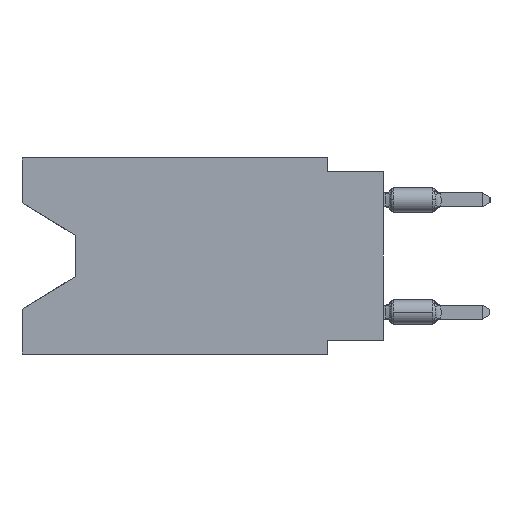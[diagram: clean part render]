
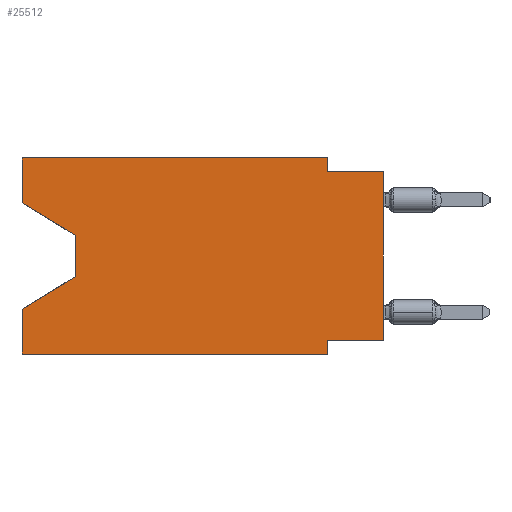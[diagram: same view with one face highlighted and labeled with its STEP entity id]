
A CAD part, left-side view. The second image highlights one B-rep face of the part: STEP entity #25512.
In plain terms, the highlighted planar face has unit normal (-1, 0, 0).
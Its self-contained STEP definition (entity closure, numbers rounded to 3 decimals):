
#20 = CARTESIAN_POINT ( 'NONE',  ( 0., 0., 0. ) ) ;
#696 = AXIS2_PLACEMENT_3D ( 'NONE', #6704, #10445, #43585 ) ;
#1336 = LINE ( 'NONE', #41915, #28280 ) ;
#2586 = VERTEX_POINT ( 'NONE', #45699 ) ;
#2714 = VERTEX_POINT ( 'NONE', #10147 ) ;
#3688 = VECTOR ( 'NONE', #42224, 1000. ) ;
#3750 = VECTOR ( 'NONE', #26880, 1000. ) ;
#3807 = EDGE_CURVE ( 'NONE', #29606, #2586, #11725, .T. ) ;
#5046 = LINE ( 'NONE', #40868, #29410 ) ;
#5248 = VECTOR ( 'NONE', #26307, 1000. ) ;
#5358 = VERTEX_POINT ( 'NONE', #15399 ) ;
#5887 = DIRECTION ( 'NONE',  ( 0., -1., 0. ) ) ;
#6704 = CARTESIAN_POINT ( 'NONE',  ( 0., 16.383, 0. ) ) ;
#6918 = ORIENTED_EDGE ( 'NONE', *, *, #27412, .F. ) ;
#7572 = ORIENTED_EDGE ( 'NONE', *, *, #3807, .T. ) ;
#9742 = VERTEX_POINT ( 'NONE', #44447 ) ;
#9893 = CARTESIAN_POINT ( 'NONE',  ( 0., 16.383, -8.89 ) ) ;
#10123 = CARTESIAN_POINT ( 'NONE',  ( 0., 0., -0.635 ) ) ;
#10147 = CARTESIAN_POINT ( 'NONE',  ( 0., 0., -8.255 ) ) ;
#10445 = DIRECTION ( 'NONE',  ( 1., 0., 0. ) ) ;
#11347 = CARTESIAN_POINT ( 'NONE',  ( 0., 16.383, -2.038 ) ) ;
#11725 = LINE ( 'NONE', #23680, #15605 ) ;
#12959 = LINE ( 'NONE', #29158, #32924 ) ;
#14047 = EDGE_CURVE ( 'NONE', #5358, #40531, #46461, .T. ) ;
#14627 = VECTOR ( 'NONE', #35396, 1000. ) ;
#14954 = EDGE_CURVE ( 'NONE', #45347, #30562, #18975, .T. ) ;
#15399 = CARTESIAN_POINT ( 'NONE',  ( 0., 2.54, -0.635 ) ) ;
#15605 = VECTOR ( 'NONE', #39050, 1000. ) ;
#15626 = VECTOR ( 'NONE', #34856, 1000. ) ;
#15962 = LINE ( 'NONE', #20, #33531 ) ;
#15999 = ORIENTED_EDGE ( 'NONE', *, *, #28904, .T. ) ;
#16475 = VERTEX_POINT ( 'NONE', #50000 ) ;
#16602 = EDGE_CURVE ( 'NONE', #50305, #16475, #51574, .T. ) ;
#16697 = CARTESIAN_POINT ( 'NONE',  ( 0., 2.54, -8.89 ) ) ;
#18657 = PLANE ( 'NONE',  #696 ) ;
#18975 = LINE ( 'NONE', #39366, #14627 ) ;
#19158 = LINE ( 'NONE', #9893, #41328 ) ;
#23680 = CARTESIAN_POINT ( 'NONE',  ( 0., 16.383, -2.038 ) ) ;
#25512 = ADVANCED_FACE ( 'NONE', ( #31375 ), #18657, .F. ) ;
#25763 = DIRECTION ( 'NONE',  ( 0., 1., 0. ) ) ;
#25820 = ORIENTED_EDGE ( 'NONE', *, *, #14047, .F. ) ;
#26233 = EDGE_CURVE ( 'NONE', #42899, #36298, #12959, .T. ) ;
#26307 = DIRECTION ( 'NONE',  ( 0., -1., 0. ) ) ;
#26880 = DIRECTION ( 'NONE',  ( 0., 0., 1. ) ) ;
#27173 = CARTESIAN_POINT ( 'NONE',  ( 0., 16.383, 0. ) ) ;
#27412 = EDGE_CURVE ( 'NONE', #36298, #5358, #50774, .T. ) ;
#27600 = VECTOR ( 'NONE', #37721, 1000. ) ;
#27612 = EDGE_CURVE ( 'NONE', #2714, #40531, #15962, .T. ) ;
#27769 = ORIENTED_EDGE ( 'NONE', *, *, #26233, .F. ) ;
#28280 = VECTOR ( 'NONE', #25763, 1000. ) ;
#28680 = DIRECTION ( 'NONE',  ( 0., 0., 1. ) ) ;
#28904 = EDGE_CURVE ( 'NONE', #9742, #16475, #5046, .T. ) ;
#29158 = CARTESIAN_POINT ( 'NONE',  ( 0., 16.383, 0. ) ) ;
#29410 = VECTOR ( 'NONE', #41127, 1000. ) ;
#29606 = VERTEX_POINT ( 'NONE', #11347 ) ;
#30462 = CARTESIAN_POINT ( 'NONE',  ( 0., 16.383, -8.89 ) ) ;
#30562 = VERTEX_POINT ( 'NONE', #16697 ) ;
#31375 = FACE_OUTER_BOUND ( 'NONE', #42587, .T. ) ;
#32772 = CARTESIAN_POINT ( 'NONE',  ( 0., 2.54, 0. ) ) ;
#32924 = VECTOR ( 'NONE', #41070, 1000. ) ;
#33531 = VECTOR ( 'NONE', #28680, 1000. ) ;
#33952 = ORIENTED_EDGE ( 'NONE', *, *, #52446, .T. ) ;
#34593 = ORIENTED_EDGE ( 'NONE', *, *, #27612, .T. ) ;
#34856 = DIRECTION ( 'NONE',  ( 0., 0., 1. ) ) ;
#35396 = DIRECTION ( 'NONE',  ( 0., 0., -1. ) ) ;
#36298 = VERTEX_POINT ( 'NONE', #32772 ) ;
#37721 = DIRECTION ( 'NONE',  ( 0., 0., -1. ) ) ;
#37757 = ORIENTED_EDGE ( 'NONE', *, *, #14954, .F. ) ;
#38175 = ORIENTED_EDGE ( 'NONE', *, *, #16602, .F. ) ;
#38251 = CARTESIAN_POINT ( 'NONE',  ( 0., 2.54, 0. ) ) ;
#39049 = CARTESIAN_POINT ( 'NONE',  ( 0., 16.383, 0. ) ) ;
#39050 = DIRECTION ( 'NONE',  ( 0., -0.855, -0.519 ) ) ;
#39366 = CARTESIAN_POINT ( 'NONE',  ( 0., 2.54, -8.89 ) ) ;
#39550 = CARTESIAN_POINT ( 'NONE',  ( 0., 2.54, -8.255 ) ) ;
#40124 = ORIENTED_EDGE ( 'NONE', *, *, #44016, .T. ) ;
#40531 = VERTEX_POINT ( 'NONE', #41234 ) ;
#40868 = CARTESIAN_POINT ( 'NONE',  ( 0., 13.97, -5.385 ) ) ;
#41070 = DIRECTION ( 'NONE',  ( 0., -1., 0. ) ) ;
#41127 = DIRECTION ( 'NONE',  ( 0., 0.855, -0.519 ) ) ;
#41234 = CARTESIAN_POINT ( 'NONE',  ( 0., 0., -0.635 ) ) ;
#41328 = VECTOR ( 'NONE', #5887, 1000. ) ;
#41807 = ORIENTED_EDGE ( 'NONE', *, *, #46514, .F. ) ;
#41915 = CARTESIAN_POINT ( 'NONE',  ( 0., 0., -8.255 ) ) ;
#42224 = DIRECTION ( 'NONE',  ( 0., 0., -1. ) ) ;
#42587 = EDGE_LOOP ( 'NONE', ( #7572, #40124, #15999, #38175, #33952, #37757, #44048, #34593, #25820, #6918, #27769, #41807 ) ) ;
#42899 = VERTEX_POINT ( 'NONE', #50749 ) ;
#43585 = DIRECTION ( 'NONE',  ( 0., 0., -1. ) ) ;
#44016 = EDGE_CURVE ( 'NONE', #2586, #9742, #50498, .T. ) ;
#44048 = ORIENTED_EDGE ( 'NONE', *, *, #45619, .F. ) ;
#44447 = CARTESIAN_POINT ( 'NONE',  ( 0., 13.97, -5.385 ) ) ;
#45347 = VERTEX_POINT ( 'NONE', #39550 ) ;
#45619 = EDGE_CURVE ( 'NONE', #2714, #45347, #1336, .T. ) ;
#45699 = CARTESIAN_POINT ( 'NONE',  ( 0., 13.97, -3.505 ) ) ;
#45974 = CARTESIAN_POINT ( 'NONE',  ( 0., 13.97, -3.505 ) ) ;
#46461 = LINE ( 'NONE', #10123, #5248 ) ;
#46514 = EDGE_CURVE ( 'NONE', #29606, #42899, #47324, .T. ) ;
#47324 = LINE ( 'NONE', #27173, #15626 ) ;
#50000 = CARTESIAN_POINT ( 'NONE',  ( 0., 16.383, -6.852 ) ) ;
#50305 = VERTEX_POINT ( 'NONE', #30462 ) ;
#50498 = LINE ( 'NONE', #45974, #3688 ) ;
#50749 = CARTESIAN_POINT ( 'NONE',  ( 0., 16.383, 0. ) ) ;
#50774 = LINE ( 'NONE', #38251, #27600 ) ;
#51574 = LINE ( 'NONE', #39049, #3750 ) ;
#52446 = EDGE_CURVE ( 'NONE', #50305, #30562, #19158, .T. ) ;
